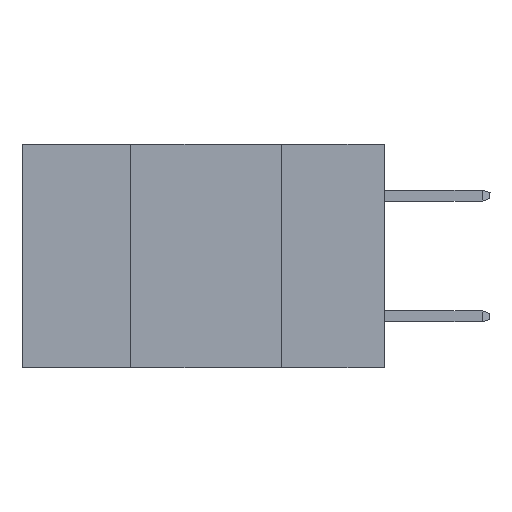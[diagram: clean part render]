
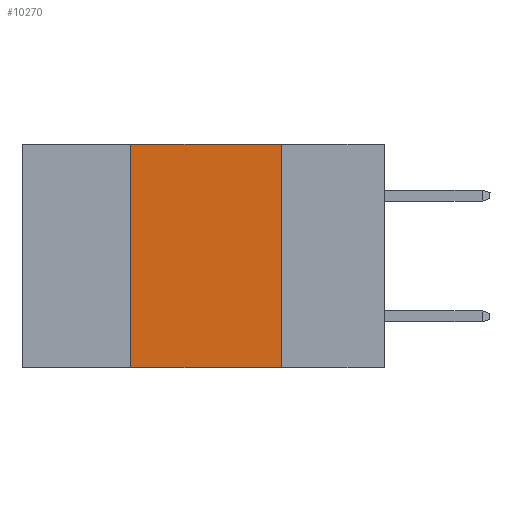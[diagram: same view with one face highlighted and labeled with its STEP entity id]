
A CAD part, left-side view. The second image highlights one B-rep face of the part: STEP entity #10270.
In plain terms, the highlighted planar face has unit normal (-1, 0, 0).
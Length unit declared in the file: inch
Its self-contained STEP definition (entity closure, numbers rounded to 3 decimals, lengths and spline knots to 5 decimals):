
#127 = LINE ( 'NONE', #375, #10642 ) ;
#375 = CARTESIAN_POINT ( 'NONE',  ( 0., 0.17, 0. ) ) ;
#895 = VECTOR ( 'NONE', #10880, 39.37008 ) ;
#1194 = AXIS2_PLACEMENT_3D ( 'NONE', #5949, #1465, #8574 ) ;
#1321 = LINE ( 'NONE', #8258, #895 ) ;
#1465 = DIRECTION ( 'NONE',  ( 1., 0., 0. ) ) ;
#1544 = EDGE_CURVE ( 'NONE', #1828, #2764, #7750, .T. ) ;
#1797 = ORIENTED_EDGE ( 'NONE', *, *, #8409, .F. ) ;
#1828 = VERTEX_POINT ( 'NONE', #9415 ) ;
#2373 = CARTESIAN_POINT ( 'NONE',  ( 0., 0.42, -0.37 ) ) ;
#2447 = DIRECTION ( 'NONE',  ( 0., -1., 0. ) ) ;
#2554 = VERTEX_POINT ( 'NONE', #2373 ) ;
#2752 = CARTESIAN_POINT ( 'NONE',  ( 0., 0.17, 0. ) ) ;
#2764 = VERTEX_POINT ( 'NONE', #2752 ) ;
#3284 = ORIENTED_EDGE ( 'NONE', *, *, #5855, .T. ) ;
#3783 = EDGE_LOOP ( 'NONE', ( #4433, #10690, #1797, #3284 ) ) ;
#4149 = PLANE ( 'NONE',  #1194 ) ;
#4433 = ORIENTED_EDGE ( 'NONE', *, *, #5256, .F. ) ;
#5256 = EDGE_CURVE ( 'NONE', #2764, #5607, #127, .T. ) ;
#5607 = VERTEX_POINT ( 'NONE', #6597 ) ;
#5664 = LINE ( 'NONE', #6826, #7058 ) ;
#5855 = EDGE_CURVE ( 'NONE', #2554, #5607, #5664, .T. ) ;
#5949 = CARTESIAN_POINT ( 'NONE',  ( 0., 0.6, 0. ) ) ;
#6597 = CARTESIAN_POINT ( 'NONE',  ( 0., 0.17, -0.37 ) ) ;
#6826 = CARTESIAN_POINT ( 'NONE',  ( 0., 0.6, -0.37 ) ) ;
#7058 = VECTOR ( 'NONE', #2447, 39.37008 ) ;
#7750 = LINE ( 'NONE', #10742, #9791 ) ;
#8258 = CARTESIAN_POINT ( 'NONE',  ( 0., 0.42, 0. ) ) ;
#8409 = EDGE_CURVE ( 'NONE', #2554, #1828, #1321, .T. ) ;
#8574 = DIRECTION ( 'NONE',  ( 0., 0., -1. ) ) ;
#9415 = CARTESIAN_POINT ( 'NONE',  ( 0., 0.42, 0. ) ) ;
#9791 = VECTOR ( 'NONE', #10860, 39.37008 ) ;
#10043 = DIRECTION ( 'NONE',  ( 0., 0., -1. ) ) ;
#10270 = ADVANCED_FACE ( 'NONE', ( #11252 ), #4149, .F. ) ;
#10642 = VECTOR ( 'NONE', #10043, 39.37008 ) ;
#10690 = ORIENTED_EDGE ( 'NONE', *, *, #1544, .F. ) ;
#10742 = CARTESIAN_POINT ( 'NONE',  ( 0., 0.6, 0. ) ) ;
#10860 = DIRECTION ( 'NONE',  ( 0., -1., 0. ) ) ;
#10880 = DIRECTION ( 'NONE',  ( 0., 0., 1. ) ) ;
#11252 = FACE_OUTER_BOUND ( 'NONE', #3783, .T. ) ;
